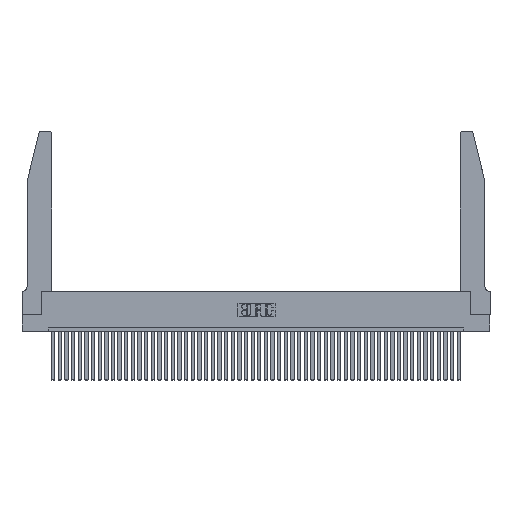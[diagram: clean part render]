
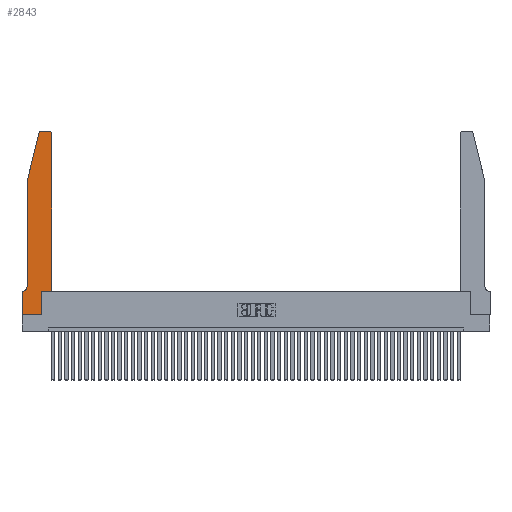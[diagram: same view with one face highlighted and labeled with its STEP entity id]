
A CAD part, top view. The second image highlights one B-rep face of the part: STEP entity #2843.
In plain terms, the highlighted planar face has unit normal (0, 0, 1).
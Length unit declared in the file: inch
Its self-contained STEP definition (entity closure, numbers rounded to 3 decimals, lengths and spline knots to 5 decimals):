
#974 = VERTEX_POINT ( 'NONE', #12812 ) ;
#1038 = LINE ( 'NONE', #36523, #39845 ) ;
#1537 = CARTESIAN_POINT ( 'NONE',  ( 0.2865, 0., 0.37 ) ) ;
#1743 = DIRECTION ( 'NONE',  ( 1., 0., 0. ) ) ;
#1827 = CARTESIAN_POINT ( 'NONE',  ( 0.0755, 2., 0.37 ) ) ;
#2170 = CARTESIAN_POINT ( 'NONE',  ( 0.0755, 2., 0.37 ) ) ;
#2564 = AXIS2_PLACEMENT_3D ( 'NONE', #7413, #29680, #33938 ) ;
#2843 = ADVANCED_FACE ( 'NONE', ( #11604 ), #4597, .T. ) ;
#3147 = DIRECTION ( 'NONE',  ( -0.239, -0.971, 0. ) ) ;
#4054 = EDGE_CURVE ( 'NONE', #974, #29065, #11421, .T. ) ;
#4070 = LINE ( 'NONE', #15851, #16415 ) ;
#4597 = PLANE ( 'NONE',  #20451 ) ;
#4887 = DIRECTION ( 'NONE',  ( 0., -1., 0. ) ) ;
#5013 = DIRECTION ( 'NONE',  ( -1., 0., 0. ) ) ;
#5208 = ORIENTED_EDGE ( 'NONE', *, *, #12147, .T. ) ;
#5749 = CIRCLE ( 'NONE', #12733, 0.07 ) ;
#5896 = VECTOR ( 'NONE', #3147, 39.37008 ) ;
#6660 = DIRECTION ( 'NONE',  ( -1., 0., 0. ) ) ;
#6703 = LINE ( 'NONE', #7965, #36061 ) ;
#7106 = CARTESIAN_POINT ( 'NONE',  ( 0.0055, 0.42, 0.37 ) ) ;
#7213 = ORIENTED_EDGE ( 'NONE', *, *, #11397, .T. ) ;
#7413 = CARTESIAN_POINT ( 'NONE',  ( 0.4205, 2.72, 0.37 ) ) ;
#7965 = CARTESIAN_POINT ( 'NONE',  ( 0.2865, 0.35, 0.37 ) ) ;
#8162 = CARTESIAN_POINT ( 'NONE',  ( 0.0755, 0.42, 0.37 ) ) ;
#8258 = EDGE_CURVE ( 'NONE', #38915, #39945, #5749, .T. ) ;
#8593 = DIRECTION ( 'NONE',  ( 1., 0., 0. ) ) ;
#9012 = ORIENTED_EDGE ( 'NONE', *, *, #33187, .T. ) ;
#9097 = CARTESIAN_POINT ( 'NONE',  ( 0.4505, 0.35, 0.37 ) ) ;
#10229 = VERTEX_POINT ( 'NONE', #40092 ) ;
#10575 = LINE ( 'NONE', #23540, #36385 ) ;
#11087 = AXIS2_PLACEMENT_3D ( 'NONE', #45913, #46236, #31128 ) ;
#11397 = EDGE_CURVE ( 'NONE', #29106, #38915, #10575, .T. ) ;
#11421 = CIRCLE ( 'NONE', #2564, 0.03 ) ;
#11604 = FACE_OUTER_BOUND ( 'NONE', #48448, .T. ) ;
#11965 = CARTESIAN_POINT ( 'NONE',  ( 0., 0.35, 0.37 ) ) ;
#12147 = EDGE_CURVE ( 'NONE', #39945, #33755, #1038, .T. ) ;
#12666 = CARTESIAN_POINT ( 'NONE',  ( 0., 0., 0.37 ) ) ;
#12733 = AXIS2_PLACEMENT_3D ( 'NONE', #7106, #37108, #18433 ) ;
#12812 = CARTESIAN_POINT ( 'NONE',  ( 0.4505, 2.72, 0.37 ) ) ;
#13200 = VERTEX_POINT ( 'NONE', #12666 ) ;
#13622 = ORIENTED_EDGE ( 'NONE', *, *, #44655, .T. ) ;
#14176 = LINE ( 'NONE', #2170, #5896 ) ;
#15336 = CARTESIAN_POINT ( 'NONE',  ( 0.4505, 0.35, 0.37 ) ) ;
#15571 = ORIENTED_EDGE ( 'NONE', *, *, #8258, .T. ) ;
#15765 = DIRECTION ( 'NONE',  ( 0., 0., 1. ) ) ;
#15767 = CARTESIAN_POINT ( 'NONE',  ( 0.4205, 2.75, 0.37 ) ) ;
#15851 = CARTESIAN_POINT ( 'NONE',  ( 0.4505, 0.35, 0.37 ) ) ;
#16083 = ORIENTED_EDGE ( 'NONE', *, *, #21381, .T. ) ;
#16141 = VERTEX_POINT ( 'NONE', #9097 ) ;
#16360 = DIRECTION ( 'NONE',  ( 0., -1., 0. ) ) ;
#16415 = VECTOR ( 'NONE', #8593, 39.37008 ) ;
#18433 = DIRECTION ( 'NONE',  ( -1., 0., 0. ) ) ;
#19664 = VECTOR ( 'NONE', #4887, 39.37008 ) ;
#20407 = ORIENTED_EDGE ( 'NONE', *, *, #33360, .T. ) ;
#20451 = AXIS2_PLACEMENT_3D ( 'NONE', #11965, #15765, #30788 ) ;
#20867 = ORIENTED_EDGE ( 'NONE', *, *, #37953, .T. ) ;
#21061 = CARTESIAN_POINT ( 'NONE',  ( 0., 0.35, 0.37 ) ) ;
#21381 = EDGE_CURVE ( 'NONE', #33755, #13200, #25587, .T. ) ;
#21689 = CARTESIAN_POINT ( 'NONE',  ( 0.284, 2.75, 0.37 ) ) ;
#22911 = DIRECTION ( 'NONE',  ( 0., 1., 0. ) ) ;
#23540 = CARTESIAN_POINT ( 'NONE',  ( 0.0755, 2., 0.37 ) ) ;
#23748 = CARTESIAN_POINT ( 'NONE',  ( 0., 0., 0.37 ) ) ;
#23799 = VECTOR ( 'NONE', #40898, 39.37008 ) ;
#24419 = LINE ( 'NONE', #15336, #23799 ) ;
#25465 = LINE ( 'NONE', #34853, #34219 ) ;
#25587 = LINE ( 'NONE', #23748, #19664 ) ;
#26786 = VECTOR ( 'NONE', #1743, 39.37008 ) ;
#29065 = VERTEX_POINT ( 'NONE', #15767 ) ;
#29106 = VERTEX_POINT ( 'NONE', #1827 ) ;
#29680 = DIRECTION ( 'NONE',  ( 0., 0., 1. ) ) ;
#30788 = DIRECTION ( 'NONE',  ( 1., 0., 0. ) ) ;
#31128 = DIRECTION ( 'NONE',  ( 1., 0., 0. ) ) ;
#31163 = CARTESIAN_POINT ( 'NONE',  ( 0.25487, 2.72718, 0.37 ) ) ;
#33174 = ORIENTED_EDGE ( 'NONE', *, *, #35050, .T. ) ;
#33187 = EDGE_CURVE ( 'NONE', #47419, #48451, #41626, .T. ) ;
#33360 = EDGE_CURVE ( 'NONE', #48451, #29106, #14176, .T. ) ;
#33755 = VERTEX_POINT ( 'NONE', #21061 ) ;
#33938 = DIRECTION ( 'NONE',  ( 1., 0., 0. ) ) ;
#33995 = CARTESIAN_POINT ( 'NONE',  ( 0.0055, 0.35, 0.37 ) ) ;
#34219 = VECTOR ( 'NONE', #5013, 39.37008 ) ;
#34853 = CARTESIAN_POINT ( 'NONE',  ( 0.2605, 2.75, 0.37 ) ) ;
#35050 = EDGE_CURVE ( 'NONE', #29065, #47419, #25465, .T. ) ;
#35098 = ORIENTED_EDGE ( 'NONE', *, *, #4054, .T. ) ;
#36061 = VECTOR ( 'NONE', #22911, 39.37008 ) ;
#36385 = VECTOR ( 'NONE', #16360, 39.37008 ) ;
#36523 = CARTESIAN_POINT ( 'NONE',  ( 0.0755, 0.35, 0.37 ) ) ;
#37108 = DIRECTION ( 'NONE',  ( 0., 0., -1. ) ) ;
#37953 = EDGE_CURVE ( 'NONE', #10229, #16141, #4070, .T. ) ;
#38915 = VERTEX_POINT ( 'NONE', #8162 ) ;
#39845 = VECTOR ( 'NONE', #6660, 39.37008 ) ;
#39945 = VERTEX_POINT ( 'NONE', #33995 ) ;
#39967 = EDGE_CURVE ( 'NONE', #16141, #974, #24419, .T. ) ;
#39984 = ORIENTED_EDGE ( 'NONE', *, *, #39967, .T. ) ;
#40092 = CARTESIAN_POINT ( 'NONE',  ( 0.2865, 0.35, 0.37 ) ) ;
#40898 = DIRECTION ( 'NONE',  ( 0., 1., 0. ) ) ;
#41626 = CIRCLE ( 'NONE', #11087, 0.03 ) ;
#42500 = EDGE_CURVE ( 'NONE', #13200, #43659, #48000, .T. ) ;
#43659 = VERTEX_POINT ( 'NONE', #1537 ) ;
#44655 = EDGE_CURVE ( 'NONE', #43659, #10229, #6703, .T. ) ;
#45913 = CARTESIAN_POINT ( 'NONE',  ( 0.284, 2.72, 0.37 ) ) ;
#46236 = DIRECTION ( 'NONE',  ( 0., 0., 1. ) ) ;
#46997 = CARTESIAN_POINT ( 'NONE',  ( 0., 0., 0.37 ) ) ;
#47256 = ORIENTED_EDGE ( 'NONE', *, *, #42500, .T. ) ;
#47419 = VERTEX_POINT ( 'NONE', #21689 ) ;
#48000 = LINE ( 'NONE', #46997, #26786 ) ;
#48448 = EDGE_LOOP ( 'NONE', ( #33174, #9012, #20407, #7213, #15571, #5208, #16083, #47256, #13622, #20867, #39984, #35098 ) ) ;
#48451 = VERTEX_POINT ( 'NONE', #31163 ) ;
